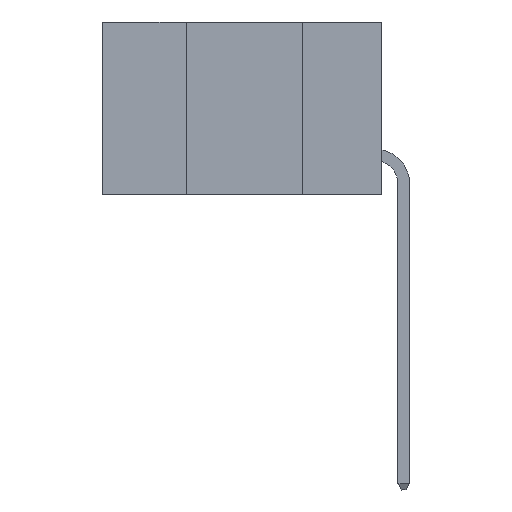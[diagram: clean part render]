
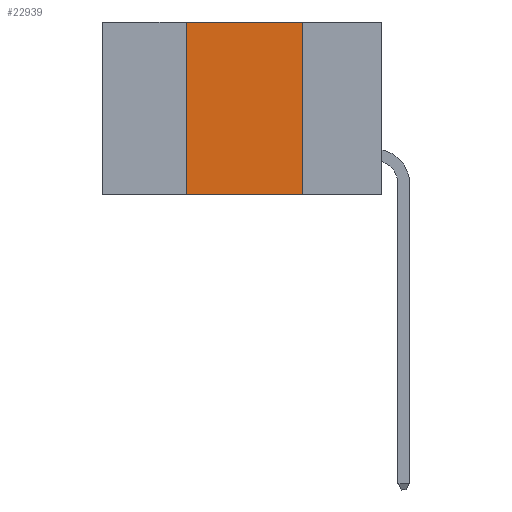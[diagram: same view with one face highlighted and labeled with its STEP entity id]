
A CAD part, left-side view. The second image highlights one B-rep face of the part: STEP entity #22939.
In plain terms, the highlighted planar face has unit normal (-1, 0, 0).
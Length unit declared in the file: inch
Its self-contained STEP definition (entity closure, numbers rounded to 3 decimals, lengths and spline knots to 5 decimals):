
#96 = VECTOR ( 'NONE', #10535, 39.37008 ) ;
#928 = CARTESIAN_POINT ( 'NONE',  ( 0., 0.6, 0. ) ) ;
#972 = EDGE_CURVE ( 'NONE', #20796, #1937, #15988, .T. ) ;
#1509 = EDGE_CURVE ( 'NONE', #13158, #20796, #17978, .T. ) ;
#1937 = VERTEX_POINT ( 'NONE', #15452 ) ;
#2015 = CARTESIAN_POINT ( 'NONE',  ( 0., 0.6, 0. ) ) ;
#2752 = CARTESIAN_POINT ( 'NONE',  ( 0., 0.42, 0. ) ) ;
#2929 = CARTESIAN_POINT ( 'NONE',  ( 0., 0.42, -0.37 ) ) ;
#4455 = FACE_OUTER_BOUND ( 'NONE', #6822, .T. ) ;
#4506 = DIRECTION ( 'NONE',  ( 0., 0., 1. ) ) ;
#4760 = ORIENTED_EDGE ( 'NONE', *, *, #14923, .F. ) ;
#6334 = CARTESIAN_POINT ( 'NONE',  ( 0., 0.17, 0. ) ) ;
#6393 = CARTESIAN_POINT ( 'NONE',  ( 0., 0.42, 0. ) ) ;
#6822 = EDGE_LOOP ( 'NONE', ( #4760, #10551, #9584, #21421 ) ) ;
#8123 = DIRECTION ( 'NONE',  ( 0., 0., -1. ) ) ;
#8396 = DIRECTION ( 'NONE',  ( 0., -1., 0. ) ) ;
#8797 = CARTESIAN_POINT ( 'NONE',  ( 0., 0.6, -0.37 ) ) ;
#9584 = ORIENTED_EDGE ( 'NONE', *, *, #1509, .F. ) ;
#9776 = LINE ( 'NONE', #8797, #96 ) ;
#10535 = DIRECTION ( 'NONE',  ( 0., -1., 0. ) ) ;
#10551 = ORIENTED_EDGE ( 'NONE', *, *, #972, .F. ) ;
#10793 = VECTOR ( 'NONE', #8396, 39.37008 ) ;
#10946 = DIRECTION ( 'NONE',  ( 0., 0., -1. ) ) ;
#12897 = VERTEX_POINT ( 'NONE', #16299 ) ;
#13143 = VECTOR ( 'NONE', #4506, 39.37008 ) ;
#13158 = VERTEX_POINT ( 'NONE', #2929 ) ;
#14726 = AXIS2_PLACEMENT_3D ( 'NONE', #2015, #21595, #10946 ) ;
#14923 = EDGE_CURVE ( 'NONE', #1937, #12897, #16117, .T. ) ;
#15452 = CARTESIAN_POINT ( 'NONE',  ( 0., 0.17, 0. ) ) ;
#15988 = LINE ( 'NONE', #928, #10793 ) ;
#16117 = LINE ( 'NONE', #6334, #20373 ) ;
#16299 = CARTESIAN_POINT ( 'NONE',  ( 0., 0.17, -0.37 ) ) ;
#17978 = LINE ( 'NONE', #2752, #13143 ) ;
#18121 = EDGE_CURVE ( 'NONE', #13158, #12897, #9776, .T. ) ;
#19811 = PLANE ( 'NONE',  #14726 ) ;
#20373 = VECTOR ( 'NONE', #8123, 39.37008 ) ;
#20796 = VERTEX_POINT ( 'NONE', #6393 ) ;
#21421 = ORIENTED_EDGE ( 'NONE', *, *, #18121, .T. ) ;
#21595 = DIRECTION ( 'NONE',  ( 1., 0., 0. ) ) ;
#22939 = ADVANCED_FACE ( 'NONE', ( #4455 ), #19811, .F. ) ;
